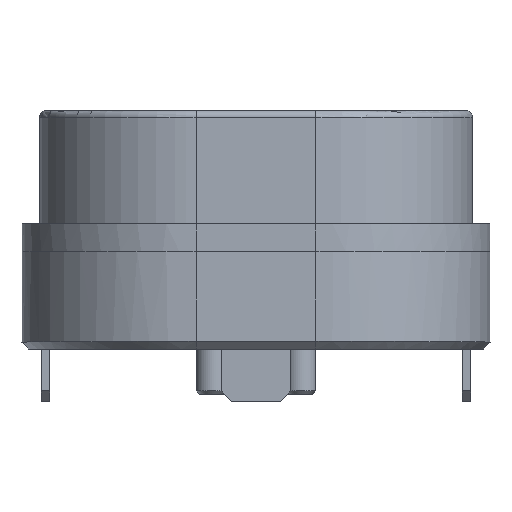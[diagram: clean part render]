
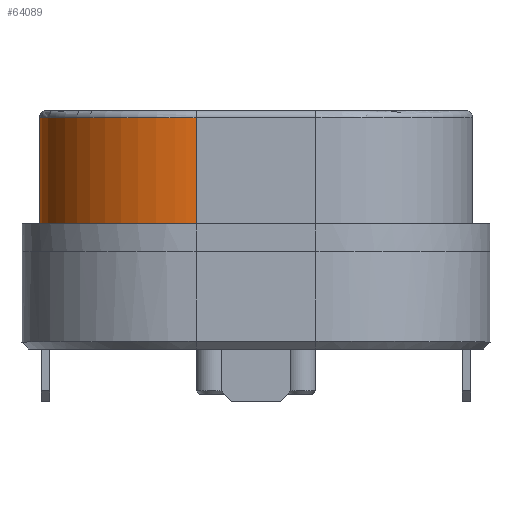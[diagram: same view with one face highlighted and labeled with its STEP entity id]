
A CAD part, left-side view. The second image highlights one B-rep face of the part: STEP entity #64089.
In plain terms, the highlighted cylindrical face has radius 4.5 mm (diameter 9 mm), a partial arc.
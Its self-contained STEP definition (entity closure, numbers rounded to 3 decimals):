
#400 = VERTEX_POINT ( 'NONE', #61754 ) ;
#453 = CARTESIAN_POINT ( 'NONE',  ( -163.69, -48.28, -1.017 ) ) ;
#3919 = CARTESIAN_POINT ( 'NONE',  ( -163.69, -48.28, -3.05 ) ) ;
#4816 = VERTEX_POINT ( 'NONE', #19162 ) ;
#5095 = CARTESIAN_POINT ( 'NONE',  ( -163.69, -48.28, -2.033 ) ) ;
#6513 = ORIENTED_EDGE ( 'NONE', *, *, #32744, .F. ) ;
#6531 = CARTESIAN_POINT ( 'NONE',  ( -159.19, -43.78, -3.05 ) ) ;
#6923 = DIRECTION ( 'NONE',  ( 1., 0., 0. ) ) ;
#8197 = CARTESIAN_POINT ( 'NONE',  ( -161.955, -44.681, -3.05 ) ) ;
#8824 = CARTESIAN_POINT ( 'NONE',  ( -163.69, -47.691, -3.05 ) ) ;
#10081 = CARTESIAN_POINT ( 'NONE',  ( -163.573, -47.102, 0. ) ) ;
#10293 = EDGE_LOOP ( 'NONE', ( #44209, #6513, #46948, #62427 ) ) ;
#10714 = CARTESIAN_POINT ( 'NONE',  ( -163.69, -47.691, 0. ) ) ;
#10858 = CARTESIAN_POINT ( 'NONE',  ( -159.19, -48.28, -3.111 ) ) ;
#14438 = CARTESIAN_POINT ( 'NONE',  ( -160.368, -43.897, -3.05 ) ) ;
#19162 = CARTESIAN_POINT ( 'NONE',  ( -163.69, -48.28, -3.05 ) ) ;
#20982 = CARTESIAN_POINT ( 'NONE',  ( -161.955, -44.681, 0. ) ) ;
#22587 = EDGE_CURVE ( 'NONE', #4816, #400, #57217, .T. ) ;
#23377 = CARTESIAN_POINT ( 'NONE',  ( -162.789, -45.515, -3.05 ) ) ;
#26310 = CARTESIAN_POINT ( 'NONE',  ( -159.19, -43.78, 0. ) ) ;
#30375 = EDGE_CURVE ( 'NONE', #57345, #55836, #52517, .T. ) ;
#30405 = FACE_OUTER_BOUND ( 'NONE', #10293, .T. ) ;
#30592 = CARTESIAN_POINT ( 'NONE',  ( -162.789, -45.515, 0. ) ) ;
#30906 = CARTESIAN_POINT ( 'NONE',  ( -159.779, -43.78, 0. ) ) ;
#32744 = EDGE_CURVE ( 'NONE', #57345, #400, #52510, .T. ) ;
#33971 = CARTESIAN_POINT ( 'NONE',  ( -159.779, -43.78, -3.05 ) ) ;
#35211 = CARTESIAN_POINT ( 'NONE',  ( -163.122, -46.014, 0. ) ) ;
#36168 = CARTESIAN_POINT ( 'NONE',  ( -159.19, -43.78, 0. ) ) ;
#37314 = DIRECTION ( 'NONE',  ( 0., 0., 1. ) ) ;
#39556 = CARTESIAN_POINT ( 'NONE',  ( -161.456, -44.348, -3.05 ) ) ;
#42459 = CARTESIAN_POINT ( 'NONE',  ( -159.19, -43.78, -3.05 ) ) ;
#44209 = ORIENTED_EDGE ( 'NONE', *, *, #22587, .T. ) ;
#44416 = AXIS2_PLACEMENT_3D ( 'NONE', #10858, #37314, #6923 ) ;
#45799 = CARTESIAN_POINT ( 'NONE',  ( -159.19, -43.78, 0. ) ) ;
#46517 = CARTESIAN_POINT ( 'NONE',  ( -159.19, -43.78, -1.017 ) ) ;
#46948 = ORIENTED_EDGE ( 'NONE', *, *, #30375, .T. ) ;
#49180 = CARTESIAN_POINT ( 'NONE',  ( -159.19, -43.78, -3.05 ) ) ;
#49842 = CARTESIAN_POINT ( 'NONE',  ( -163.573, -47.102, -3.05 ) ) ;
#50431 = CARTESIAN_POINT ( 'NONE',  ( -163.69, -48.28, 0. ) ) ;
#50596 = CYLINDRICAL_SURFACE ( 'NONE', #44416, 4.5 ) ;
#51840 = CARTESIAN_POINT ( 'NONE',  ( -159.19, -43.78, -2.033 ) ) ;
#52510 = B_SPLINE_CURVE_WITH_KNOTS ( 'NONE', 3,
 ( #45799, #30906, #65357, #61404, #20982, #30592, #35211, #10081, #10714, #50431 ),
 .UNSPECIFIED., .F., .F.,
 ( 4, 2, 2, 2, 4 ),
 ( 0., 0.25, 0.5, 0.75, 1. ),
 .UNSPECIFIED. ) ;
#52517 = B_SPLINE_CURVE_WITH_KNOTS ( 'NONE', 3,
 ( #26310, #46517, #51840, #6531 ),
 .UNSPECIFIED., .F., .F.,
 ( 4, 4 ),
 ( 0., 1. ),
 .UNSPECIFIED. ) ;
#55341 = CARTESIAN_POINT ( 'NONE',  ( -163.69, -48.28, -3.05 ) ) ;
#55836 = VERTEX_POINT ( 'NONE', #42459 ) ;
#57217 = B_SPLINE_CURVE_WITH_KNOTS ( 'NONE', 3,
 ( #55341, #5095, #453, #64658 ),
 .UNSPECIFIED., .F., .F.,
 ( 4, 4 ),
 ( 0., 1. ),
 .UNSPECIFIED. ) ;
#57345 = VERTEX_POINT ( 'NONE', #36168 ) ;
#61034 = B_SPLINE_CURVE_WITH_KNOTS ( 'NONE', 3,
 ( #49180, #33971, #14438, #39556, #8197, #23377, #64140, #49842, #8824, #3919 ),
 .UNSPECIFIED., .F., .F.,
 ( 4, 2, 2, 2, 4 ),
 ( 0., 0.25, 0.5, 0.75, 1. ),
 .UNSPECIFIED. ) ;
#61285 = EDGE_CURVE ( 'NONE', #55836, #4816, #61034, .T. ) ;
#61404 = CARTESIAN_POINT ( 'NONE',  ( -161.456, -44.348, 0. ) ) ;
#61754 = CARTESIAN_POINT ( 'NONE',  ( -163.69, -48.28, 0. ) ) ;
#62427 = ORIENTED_EDGE ( 'NONE', *, *, #61285, .T. ) ;
#64089 = ADVANCED_FACE ( 'NONE', ( #30405 ), #50596, .T. ) ;
#64140 = CARTESIAN_POINT ( 'NONE',  ( -163.122, -46.014, -3.05 ) ) ;
#64658 = CARTESIAN_POINT ( 'NONE',  ( -163.69, -48.28, 0. ) ) ;
#65357 = CARTESIAN_POINT ( 'NONE',  ( -160.368, -43.897, 0. ) ) ;
